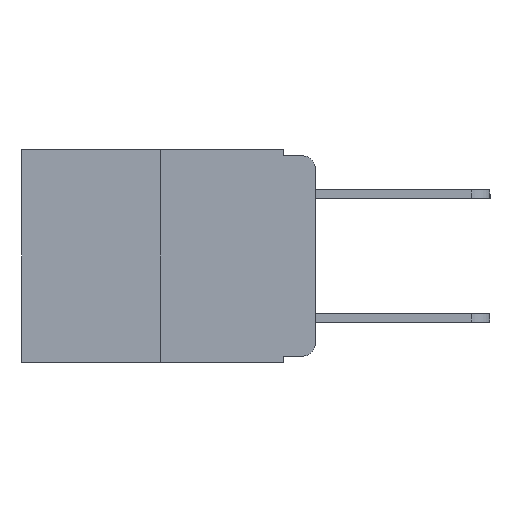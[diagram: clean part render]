
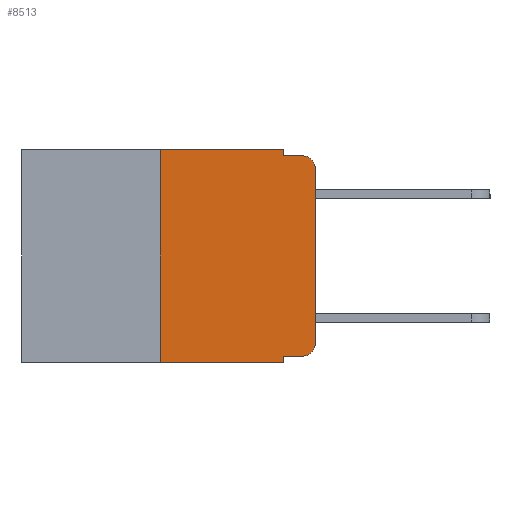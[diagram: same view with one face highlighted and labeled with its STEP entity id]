
A CAD part, left-side view. The second image highlights one B-rep face of the part: STEP entity #8513.
In plain terms, the highlighted planar face has unit normal (-1, 0, 0).
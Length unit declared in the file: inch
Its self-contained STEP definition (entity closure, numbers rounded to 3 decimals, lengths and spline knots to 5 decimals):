
#254 = EDGE_CURVE ( 'NONE', #19168, #20261, #2874, .T. ) ;
#756 = ORIENTED_EDGE ( 'NONE', *, *, #7305, .F. ) ;
#1185 = DIRECTION ( 'NONE',  ( 0., -1., 0. ) ) ;
#1526 = LINE ( 'NONE', #16332, #10867 ) ;
#1651 = CARTESIAN_POINT ( 'NONE',  ( 0., 0.051, -0.333 ) ) ;
#2302 = LINE ( 'NONE', #1651, #5914 ) ;
#2738 = VERTEX_POINT ( 'NONE', #3644 ) ;
#2872 = AXIS2_PLACEMENT_3D ( 'NONE', #18497, #8262, #20184 ) ;
#2874 = LINE ( 'NONE', #13906, #11607 ) ;
#3104 = VERTEX_POINT ( 'NONE', #17503 ) ;
#3345 = VERTEX_POINT ( 'NONE', #15261 ) ;
#3474 = DIRECTION ( 'NONE',  ( 0., 0., -1. ) ) ;
#3644 = CARTESIAN_POINT ( 'NONE',  ( 0., 0.051, 0. ) ) ;
#4853 = ORIENTED_EDGE ( 'NONE', *, *, #16376, .T. ) ;
#4856 = EDGE_CURVE ( 'NONE', #7186, #14363, #10329, .T. ) ;
#4920 = VECTOR ( 'NONE', #15511, 39.37008 ) ;
#5193 = CARTESIAN_POINT ( 'NONE',  ( 0., 0., 0. ) ) ;
#5280 = EDGE_CURVE ( 'NONE', #20263, #14363, #1526, .T. ) ;
#5914 = VECTOR ( 'NONE', #10469, 39.37008 ) ;
#5978 = CIRCLE ( 'NONE', #21124, 0.02 ) ;
#6094 = ORIENTED_EDGE ( 'NONE', *, *, #15779, .F. ) ;
#6493 = CARTESIAN_POINT ( 'NONE',  ( 0., 0.02, -0.03 ) ) ;
#6702 = EDGE_CURVE ( 'NONE', #7186, #10953, #17491, .T. ) ;
#6813 = PLANE ( 'NONE',  #13091 ) ;
#7144 = FACE_OUTER_BOUND ( 'NONE', #9133, .T. ) ;
#7186 = VERTEX_POINT ( 'NONE', #13567 ) ;
#7305 = EDGE_CURVE ( 'NONE', #2738, #19168, #17735, .T. ) ;
#7318 = ORIENTED_EDGE ( 'NONE', *, *, #254, .F. ) ;
#7847 = VECTOR ( 'NONE', #10613, 39.37008 ) ;
#8239 = DIRECTION ( 'NONE',  ( 0., 0., -1. ) ) ;
#8262 = DIRECTION ( 'NONE',  ( -1., 0., 0. ) ) ;
#8513 = ADVANCED_FACE ( 'NONE', ( #7144 ), #6813, .F. ) ;
#8549 = DIRECTION ( 'NONE',  ( 0., 0., -1. ) ) ;
#9066 = EDGE_CURVE ( 'NONE', #3345, #3104, #14123, .T. ) ;
#9133 = EDGE_LOOP ( 'NONE', ( #12130, #14844, #7318, #756, #6094, #16024, #16834, #21333, #16874, #4853 ) ) ;
#10003 = DIRECTION ( 'NONE',  ( 0., -1., 0. ) ) ;
#10136 = CARTESIAN_POINT ( 'NONE',  ( 0., 0.473, 0. ) ) ;
#10329 = LINE ( 'NONE', #14233, #14366 ) ;
#10469 = DIRECTION ( 'NONE',  ( 0., -1., 0. ) ) ;
#10613 = DIRECTION ( 'NONE',  ( 0., 0., 1. ) ) ;
#10760 = CARTESIAN_POINT ( 'NONE',  ( 0., 0.25, 0. ) ) ;
#10867 = VECTOR ( 'NONE', #17809, 39.37008 ) ;
#10953 = VERTEX_POINT ( 'NONE', #20012 ) ;
#11607 = VECTOR ( 'NONE', #10003, 39.37008 ) ;
#11691 = CARTESIAN_POINT ( 'NONE',  ( 0., 0.473, 0. ) ) ;
#11884 = LINE ( 'NONE', #11691, #12423 ) ;
#12130 = ORIENTED_EDGE ( 'NONE', *, *, #9066, .T. ) ;
#12356 = EDGE_CURVE ( 'NONE', #20263, #15413, #2302, .T. ) ;
#12423 = VECTOR ( 'NONE', #1185, 39.37008 ) ;
#12650 = CARTESIAN_POINT ( 'NONE',  ( 0., 0.051, -0.343 ) ) ;
#12670 = CIRCLE ( 'NONE', #2872, 0.02 ) ;
#13091 = AXIS2_PLACEMENT_3D ( 'NONE', #10136, #18788, #8549 ) ;
#13196 = VECTOR ( 'NONE', #3474, 39.37008 ) ;
#13567 = CARTESIAN_POINT ( 'NONE',  ( 0., 0.25, -0.343 ) ) ;
#13906 = CARTESIAN_POINT ( 'NONE',  ( 0., 0.051, -0.01 ) ) ;
#14123 = LINE ( 'NONE', #5193, #4920 ) ;
#14233 = CARTESIAN_POINT ( 'NONE',  ( 0., 0.473, -0.343 ) ) ;
#14363 = VERTEX_POINT ( 'NONE', #12650 ) ;
#14366 = VECTOR ( 'NONE', #15768, 39.37008 ) ;
#14844 = ORIENTED_EDGE ( 'NONE', *, *, #15189, .T. ) ;
#15189 = EDGE_CURVE ( 'NONE', #3104, #20261, #5978, .T. ) ;
#15261 = CARTESIAN_POINT ( 'NONE',  ( 0., 0., -0.313 ) ) ;
#15413 = VERTEX_POINT ( 'NONE', #15669 ) ;
#15511 = DIRECTION ( 'NONE',  ( 0., 0., 1. ) ) ;
#15669 = CARTESIAN_POINT ( 'NONE',  ( 0., 0.02, -0.333 ) ) ;
#15768 = DIRECTION ( 'NONE',  ( 0., -1., 0. ) ) ;
#15779 = EDGE_CURVE ( 'NONE', #10953, #2738, #11884, .T. ) ;
#16024 = ORIENTED_EDGE ( 'NONE', *, *, #6702, .F. ) ;
#16332 = CARTESIAN_POINT ( 'NONE',  ( 0., 0.051, 0. ) ) ;
#16376 = EDGE_CURVE ( 'NONE', #15413, #3345, #12670, .T. ) ;
#16834 = ORIENTED_EDGE ( 'NONE', *, *, #4856, .T. ) ;
#16874 = ORIENTED_EDGE ( 'NONE', *, *, #12356, .T. ) ;
#17491 = LINE ( 'NONE', #10760, #7847 ) ;
#17503 = CARTESIAN_POINT ( 'NONE',  ( 0., 0., -0.03 ) ) ;
#17735 = LINE ( 'NONE', #20576, #13196 ) ;
#17809 = DIRECTION ( 'NONE',  ( 0., 0., -1. ) ) ;
#18470 = DIRECTION ( 'NONE',  ( -1., 0., 0. ) ) ;
#18497 = CARTESIAN_POINT ( 'NONE',  ( 0., 0.02, -0.313 ) ) ;
#18788 = DIRECTION ( 'NONE',  ( 1., 0., 0. ) ) ;
#19026 = CARTESIAN_POINT ( 'NONE',  ( 0., 0.051, -0.333 ) ) ;
#19168 = VERTEX_POINT ( 'NONE', #19374 ) ;
#19374 = CARTESIAN_POINT ( 'NONE',  ( 0., 0.051, -0.01 ) ) ;
#20012 = CARTESIAN_POINT ( 'NONE',  ( 0., 0.25, 0. ) ) ;
#20184 = DIRECTION ( 'NONE',  ( 0., 0., -1. ) ) ;
#20261 = VERTEX_POINT ( 'NONE', #22279 ) ;
#20263 = VERTEX_POINT ( 'NONE', #19026 ) ;
#20576 = CARTESIAN_POINT ( 'NONE',  ( 0., 0.051, 0. ) ) ;
#21124 = AXIS2_PLACEMENT_3D ( 'NONE', #6493, #18470, #8239 ) ;
#21333 = ORIENTED_EDGE ( 'NONE', *, *, #5280, .F. ) ;
#22279 = CARTESIAN_POINT ( 'NONE',  ( 0., 0.02, -0.01 ) ) ;
